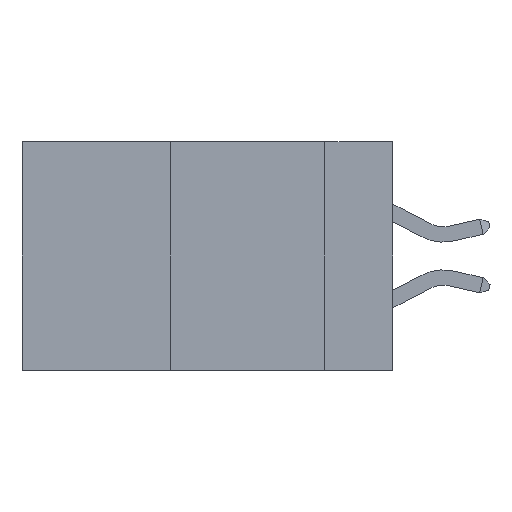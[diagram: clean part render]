
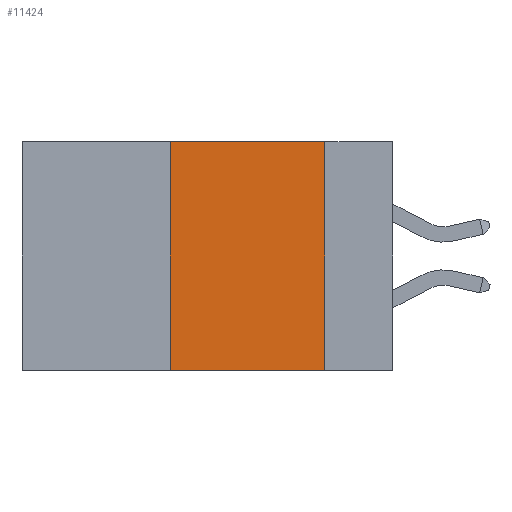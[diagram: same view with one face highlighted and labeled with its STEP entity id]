
A CAD part, left-side view. The second image highlights one B-rep face of the part: STEP entity #11424.
In plain terms, the highlighted planar face has unit normal (-1, 0, 0).
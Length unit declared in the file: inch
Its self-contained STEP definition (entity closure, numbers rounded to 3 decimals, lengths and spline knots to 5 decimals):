
#175 = ORIENTED_EDGE ( 'NONE', *, *, #13406, .F. ) ;
#1673 = VERTEX_POINT ( 'NONE', #4521 ) ;
#1733 = DIRECTION ( 'NONE',  ( 0., 0., -1. ) ) ;
#1878 = VERTEX_POINT ( 'NONE', #3590 ) ;
#2111 = VECTOR ( 'NONE', #11128, 39.37008 ) ;
#2670 = CARTESIAN_POINT ( 'NONE',  ( 0., 0.11, 0. ) ) ;
#3549 = DIRECTION ( 'NONE',  ( 0., -1., 0. ) ) ;
#3590 = CARTESIAN_POINT ( 'NONE',  ( 0., 0.36, 0. ) ) ;
#3621 = EDGE_CURVE ( 'NONE', #1673, #8368, #3922, .T. ) ;
#3922 = LINE ( 'NONE', #9563, #8599 ) ;
#4307 = DIRECTION ( 'NONE',  ( 0., 0., 1. ) ) ;
#4521 = CARTESIAN_POINT ( 'NONE',  ( 0., 0.36, -0.37 ) ) ;
#4531 = CARTESIAN_POINT ( 'NONE',  ( 0., 0.6, 0. ) ) ;
#5137 = VECTOR ( 'NONE', #11544, 39.37008 ) ;
#5491 = EDGE_LOOP ( 'NONE', ( #13127, #9792, #175, #9350 ) ) ;
#5740 = PLANE ( 'NONE',  #9457 ) ;
#5973 = LINE ( 'NONE', #8612, #11525 ) ;
#6549 = CARTESIAN_POINT ( 'NONE',  ( 0., 0.11, -0.37 ) ) ;
#7958 = LINE ( 'NONE', #13478, #5137 ) ;
#8107 = DIRECTION ( 'NONE',  ( 1., 0., 0. ) ) ;
#8368 = VERTEX_POINT ( 'NONE', #6549 ) ;
#8599 = VECTOR ( 'NONE', #3549, 39.37008 ) ;
#8612 = CARTESIAN_POINT ( 'NONE',  ( 0., 0.36, 0. ) ) ;
#9048 = EDGE_CURVE ( 'NONE', #9446, #8368, #7958, .T. ) ;
#9350 = ORIENTED_EDGE ( 'NONE', *, *, #3621, .T. ) ;
#9446 = VERTEX_POINT ( 'NONE', #2670 ) ;
#9457 = AXIS2_PLACEMENT_3D ( 'NONE', #4531, #8107, #1733 ) ;
#9563 = CARTESIAN_POINT ( 'NONE',  ( 0., 0.6, -0.37 ) ) ;
#9792 = ORIENTED_EDGE ( 'NONE', *, *, #10374, .F. ) ;
#10374 = EDGE_CURVE ( 'NONE', #1878, #9446, #12147, .T. ) ;
#11128 = DIRECTION ( 'NONE',  ( 0., -1., 0. ) ) ;
#11424 = ADVANCED_FACE ( 'NONE', ( #13604 ), #5740, .F. ) ;
#11525 = VECTOR ( 'NONE', #4307, 39.37008 ) ;
#11544 = DIRECTION ( 'NONE',  ( 0., 0., -1. ) ) ;
#12147 = LINE ( 'NONE', #13240, #2111 ) ;
#13127 = ORIENTED_EDGE ( 'NONE', *, *, #9048, .F. ) ;
#13240 = CARTESIAN_POINT ( 'NONE',  ( 0., 0.6, 0. ) ) ;
#13406 = EDGE_CURVE ( 'NONE', #1673, #1878, #5973, .T. ) ;
#13478 = CARTESIAN_POINT ( 'NONE',  ( 0., 0.11, 0. ) ) ;
#13604 = FACE_OUTER_BOUND ( 'NONE', #5491, .T. ) ;
